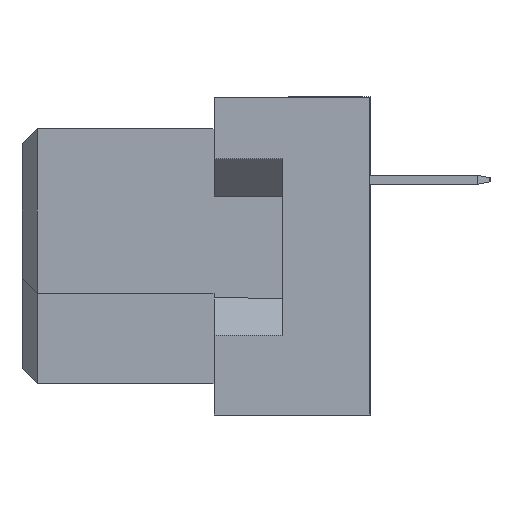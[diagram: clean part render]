
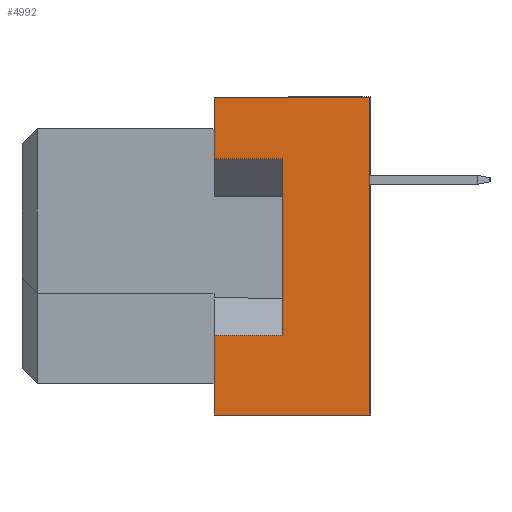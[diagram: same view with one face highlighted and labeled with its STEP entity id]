
A CAD part, left-side view. The second image highlights one B-rep face of the part: STEP entity #4992.
In plain terms, the highlighted planar face has unit normal (-1, 0, 0).
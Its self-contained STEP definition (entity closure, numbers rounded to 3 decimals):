
#57 = DIRECTION ( 'NONE',  ( 0., 0., 1. ) ) ;
#155 = DIRECTION ( 'NONE',  ( 0., 1., 0. ) ) ;
#161 = CARTESIAN_POINT ( 'NONE',  ( -27.5, -6.4, -5.3 ) ) ;
#748 = LINE ( 'NONE', #6908, #3932 ) ;
#887 = ORIENTED_EDGE ( 'NONE', *, *, #19704, .F. ) ;
#1207 = VECTOR ( 'NONE', #11832, 1000. ) ;
#1743 = LINE ( 'NONE', #16919, #5728 ) ;
#1802 = ORIENTED_EDGE ( 'NONE', *, *, #11662, .T. ) ;
#2438 = ORIENTED_EDGE ( 'NONE', *, *, #12459, .F. ) ;
#3079 = LINE ( 'NONE', #14207, #15563 ) ;
#3363 = DIRECTION ( 'NONE',  ( 0., 0., 1. ) ) ;
#3932 = VECTOR ( 'NONE', #19455, 1000. ) ;
#4056 = ORIENTED_EDGE ( 'NONE', *, *, #7564, .T. ) ;
#4531 = VERTEX_POINT ( 'NONE', #18177 ) ;
#4571 = VECTOR ( 'NONE', #155, 1000. ) ;
#4901 = VERTEX_POINT ( 'NONE', #13685 ) ;
#4992 = ADVANCED_FACE ( 'NONE', ( #15718 ), #8109, .T. ) ;
#5096 = DIRECTION ( 'NONE',  ( -1., 0., 0. ) ) ;
#5675 = LINE ( 'NONE', #6040, #18872 ) ;
#5728 = VECTOR ( 'NONE', #12561, 1000. ) ;
#5872 = ORIENTED_EDGE ( 'NONE', *, *, #15222, .F. ) ;
#6040 = CARTESIAN_POINT ( 'NONE',  ( -27.5, -6.4, -5.3 ) ) ;
#6198 = CARTESIAN_POINT ( 'NONE',  ( -27.5, -6.4, -5.3 ) ) ;
#6243 = DIRECTION ( 'NONE',  ( 0., 0., 1. ) ) ;
#6705 = CARTESIAN_POINT ( 'NONE',  ( -27.5, -11.6, 5.3 ) ) ;
#6877 = VERTEX_POINT ( 'NONE', #11528 ) ;
#6908 = CARTESIAN_POINT ( 'NONE',  ( -27.5, -8.7, 3.25 ) ) ;
#7112 = VECTOR ( 'NONE', #57, 1000. ) ;
#7382 = ORIENTED_EDGE ( 'NONE', *, *, #16814, .F. ) ;
#7564 = EDGE_CURVE ( 'NONE', #17841, #4531, #15830, .T. ) ;
#7716 = DIRECTION ( 'NONE',  ( 0., 0., 1. ) ) ;
#7922 = DIRECTION ( 'NONE',  ( 0., 1., 0. ) ) ;
#8109 = PLANE ( 'NONE',  #13204 ) ;
#8131 = LINE ( 'NONE', #17355, #4571 ) ;
#8382 = ORIENTED_EDGE ( 'NONE', *, *, #20021, .F. ) ;
#9009 = CARTESIAN_POINT ( 'NONE',  ( -27.5, -6.4, 3.25 ) ) ;
#10250 = CARTESIAN_POINT ( 'NONE',  ( -27.5, -6.4, 5.3 ) ) ;
#10692 = ORIENTED_EDGE ( 'NONE', *, *, #11768, .T. ) ;
#11528 = CARTESIAN_POINT ( 'NONE',  ( -27.5, -11.6, -5.3 ) ) ;
#11662 = EDGE_CURVE ( 'NONE', #6877, #4901, #3079, .T. ) ;
#11768 = EDGE_CURVE ( 'NONE', #4901, #11974, #8131, .T. ) ;
#11832 = DIRECTION ( 'NONE',  ( 0., 1., 0. ) ) ;
#11974 = VERTEX_POINT ( 'NONE', #10250 ) ;
#12459 = EDGE_CURVE ( 'NONE', #16918, #11974, #5675, .T. ) ;
#12561 = DIRECTION ( 'NONE',  ( 0., 0., 1. ) ) ;
#12594 = LINE ( 'NONE', #161, #7112 ) ;
#13204 = AXIS2_PLACEMENT_3D ( 'NONE', #6705, #5096, #3363 ) ;
#13685 = CARTESIAN_POINT ( 'NONE',  ( -27.5, -11.6, 5.3 ) ) ;
#14069 = VECTOR ( 'NONE', #7922, 1000. ) ;
#14207 = CARTESIAN_POINT ( 'NONE',  ( -27.5, -11.6, 5.3 ) ) ;
#15222 = EDGE_CURVE ( 'NONE', #15565, #4531, #12594, .T. ) ;
#15563 = VECTOR ( 'NONE', #7716, 1000. ) ;
#15565 = VERTEX_POINT ( 'NONE', #6198 ) ;
#15647 = CARTESIAN_POINT ( 'NONE',  ( -27.5, -8.7, -2.65 ) ) ;
#15718 = FACE_OUTER_BOUND ( 'NONE', #18059, .T. ) ;
#15830 = LINE ( 'NONE', #17038, #14069 ) ;
#16814 = EDGE_CURVE ( 'NONE', #19085, #16918, #748, .T. ) ;
#16918 = VERTEX_POINT ( 'NONE', #9009 ) ;
#16919 = CARTESIAN_POINT ( 'NONE',  ( -27.5, -8.7, -2.65 ) ) ;
#17038 = CARTESIAN_POINT ( 'NONE',  ( -27.5, -8.7, -2.65 ) ) ;
#17355 = CARTESIAN_POINT ( 'NONE',  ( -27.5, -11.6, 5.3 ) ) ;
#17841 = VERTEX_POINT ( 'NONE', #15647 ) ;
#17879 = CARTESIAN_POINT ( 'NONE',  ( -27.5, -8.7, 3.25 ) ) ;
#18059 = EDGE_LOOP ( 'NONE', ( #4056, #5872, #8382, #1802, #10692, #2438, #7382, #887 ) ) ;
#18177 = CARTESIAN_POINT ( 'NONE',  ( -27.5, -6.4, -2.65 ) ) ;
#18872 = VECTOR ( 'NONE', #6243, 1000. ) ;
#19085 = VERTEX_POINT ( 'NONE', #17879 ) ;
#19455 = DIRECTION ( 'NONE',  ( 0., 1., 0. ) ) ;
#19534 = CARTESIAN_POINT ( 'NONE',  ( -27.5, -11.6, -5.3 ) ) ;
#19630 = LINE ( 'NONE', #19534, #1207 ) ;
#19704 = EDGE_CURVE ( 'NONE', #17841, #19085, #1743, .T. ) ;
#20021 = EDGE_CURVE ( 'NONE', #6877, #15565, #19630, .T. ) ;
